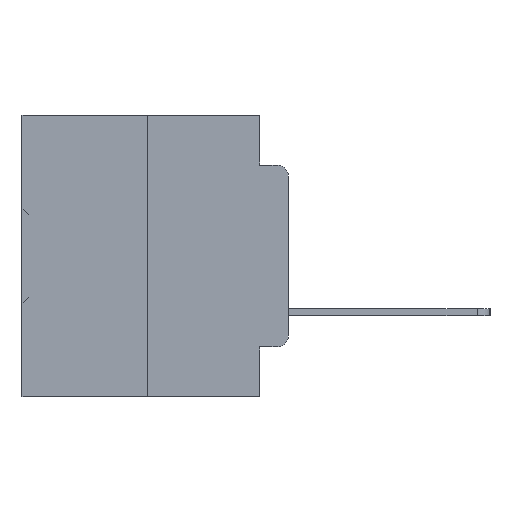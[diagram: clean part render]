
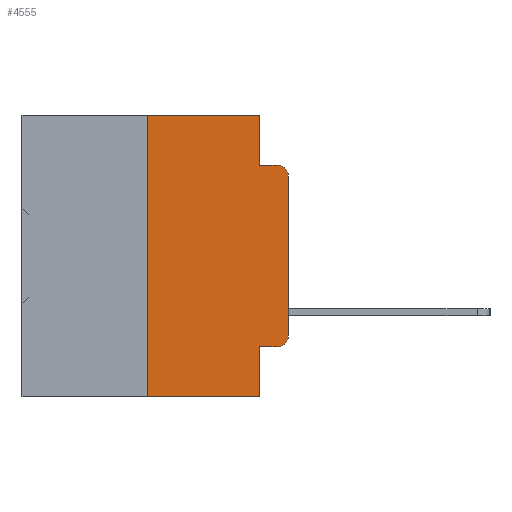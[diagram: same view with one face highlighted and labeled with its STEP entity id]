
A CAD part, left-side view. The second image highlights one B-rep face of the part: STEP entity #4555.
In plain terms, the highlighted planar face has unit normal (-1, 0, 0).
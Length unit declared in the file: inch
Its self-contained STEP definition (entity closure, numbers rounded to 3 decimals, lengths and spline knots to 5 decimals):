
#83 = CARTESIAN_POINT ( 'NONE',  ( 0., 0.25, -0.5 ) ) ;
#115 = CARTESIAN_POINT ( 'NONE',  ( 0., 0.051, -0.0885 ) ) ;
#621 = CARTESIAN_POINT ( 'NONE',  ( 0., 0.051, 0. ) ) ;
#1078 = DIRECTION ( 'NONE',  ( 0., 0., -1. ) ) ;
#1126 = DIRECTION ( 'NONE',  ( 1., 0., 0. ) ) ;
#1353 = CARTESIAN_POINT ( 'NONE',  ( 0., 0.02, -0.3915 ) ) ;
#2868 = CARTESIAN_POINT ( 'NONE',  ( 0., 0.051, -0.4115 ) ) ;
#3553 = CARTESIAN_POINT ( 'NONE',  ( 0., 0., -0.3915 ) ) ;
#3872 = ORIENTED_EDGE ( 'NONE', *, *, #26637, .F. ) ;
#4194 = FACE_OUTER_BOUND ( 'NONE', #36821, .T. ) ;
#4273 = DIRECTION ( 'NONE',  ( 0., 0., -1. ) ) ;
#4355 = DIRECTION ( 'NONE',  ( 0., -1., 0. ) ) ;
#4555 = ADVANCED_FACE ( 'NONE', ( #4194 ), #27442, .F. ) ;
#4786 = ORIENTED_EDGE ( 'NONE', *, *, #11222, .F. ) ;
#7142 = ORIENTED_EDGE ( 'NONE', *, *, #31402, .T. ) ;
#7289 = DIRECTION ( 'NONE',  ( 0., -1., 0. ) ) ;
#7305 = VECTOR ( 'NONE', #7289, 39.37008 ) ;
#7321 = EDGE_CURVE ( 'NONE', #8021, #9298, #30567, .T. ) ;
#7781 = VERTEX_POINT ( 'NONE', #17082 ) ;
#8021 = VERTEX_POINT ( 'NONE', #83 ) ;
#8659 = VERTEX_POINT ( 'NONE', #3553 ) ;
#8946 = VERTEX_POINT ( 'NONE', #2868 ) ;
#9113 = VECTOR ( 'NONE', #4355, 39.37008 ) ;
#9298 = VERTEX_POINT ( 'NONE', #10893 ) ;
#9777 = LINE ( 'NONE', #36849, #16595 ) ;
#10030 = LINE ( 'NONE', #32965, #9113 ) ;
#10893 = CARTESIAN_POINT ( 'NONE',  ( 0., 0.25, 0. ) ) ;
#11222 = EDGE_CURVE ( 'NONE', #16230, #32116, #18301, .T. ) ;
#11243 = DIRECTION ( 'NONE',  ( 0., 0., -1. ) ) ;
#11246 = ORIENTED_EDGE ( 'NONE', *, *, #7321, .F. ) ;
#11386 = CARTESIAN_POINT ( 'NONE',  ( 0., 0.02, -0.1085 ) ) ;
#12014 = AXIS2_PLACEMENT_3D ( 'NONE', #1353, #21587, #4273 ) ;
#12282 = ORIENTED_EDGE ( 'NONE', *, *, #34247, .T. ) ;
#12675 = CARTESIAN_POINT ( 'NONE',  ( 0., 0.051, 0. ) ) ;
#14001 = ORIENTED_EDGE ( 'NONE', *, *, #28544, .T. ) ;
#14309 = DIRECTION ( 'NONE',  ( 0., 0., -1. ) ) ;
#14568 = CARTESIAN_POINT ( 'NONE',  ( 0., 0.02, -0.0885 ) ) ;
#16230 = VERTEX_POINT ( 'NONE', #12675 ) ;
#16595 = VECTOR ( 'NONE', #11243, 39.37008 ) ;
#17082 = CARTESIAN_POINT ( 'NONE',  ( 0., 0.02, -0.4115 ) ) ;
#17598 = EDGE_CURVE ( 'NONE', #9298, #16230, #10030, .T. ) ;
#17795 = VERTEX_POINT ( 'NONE', #28285 ) ;
#18301 = LINE ( 'NONE', #621, #31707 ) ;
#19358 = DIRECTION ( 'NONE',  ( 0., 0., 1. ) ) ;
#19765 = VECTOR ( 'NONE', #19358, 39.37008 ) ;
#20023 = ORIENTED_EDGE ( 'NONE', *, *, #17598, .F. ) ;
#20386 = VECTOR ( 'NONE', #31371, 39.37008 ) ;
#20851 = DIRECTION ( 'NONE',  ( 0., 0., -1. ) ) ;
#21167 = LINE ( 'NONE', #35821, #27898 ) ;
#21258 = ORIENTED_EDGE ( 'NONE', *, *, #34949, .F. ) ;
#21281 = LINE ( 'NONE', #25665, #20386 ) ;
#21587 = DIRECTION ( 'NONE',  ( -1., 0., 0. ) ) ;
#22149 = VERTEX_POINT ( 'NONE', #14568 ) ;
#23080 = ORIENTED_EDGE ( 'NONE', *, *, #25427, .T. ) ;
#24493 = DIRECTION ( 'NONE',  ( 0., -1., 0. ) ) ;
#24547 = CARTESIAN_POINT ( 'NONE',  ( 0., 0.051, -0.4115 ) ) ;
#25427 = EDGE_CURVE ( 'NONE', #7781, #8659, #30842, .T. ) ;
#25665 = CARTESIAN_POINT ( 'NONE',  ( 0., 0.473, -0.5 ) ) ;
#26637 = EDGE_CURVE ( 'NONE', #32116, #22149, #21167, .T. ) ;
#27442 = PLANE ( 'NONE',  #29269 ) ;
#27898 = VECTOR ( 'NONE', #24493, 39.37008 ) ;
#28070 = CARTESIAN_POINT ( 'NONE',  ( 0., 0.473, 0. ) ) ;
#28285 = CARTESIAN_POINT ( 'NONE',  ( 0., 0.051, -0.5 ) ) ;
#28544 = EDGE_CURVE ( 'NONE', #32725, #22149, #37073, .T. ) ;
#29170 = LINE ( 'NONE', #33805, #19765 ) ;
#29269 = AXIS2_PLACEMENT_3D ( 'NONE', #28070, #1126, #1078 ) ;
#29324 = LINE ( 'NONE', #24547, #7305 ) ;
#30567 = LINE ( 'NONE', #36111, #37217 ) ;
#30842 = CIRCLE ( 'NONE', #12014, 0.02 ) ;
#31131 = EDGE_CURVE ( 'NONE', #8946, #7781, #29324, .T. ) ;
#31371 = DIRECTION ( 'NONE',  ( 0., -1., 0. ) ) ;
#31402 = EDGE_CURVE ( 'NONE', #8021, #17795, #21281, .T. ) ;
#31426 = DIRECTION ( 'NONE',  ( -1., 0., 0. ) ) ;
#31707 = VECTOR ( 'NONE', #20851, 39.37008 ) ;
#31769 = AXIS2_PLACEMENT_3D ( 'NONE', #11386, #31426, #14309 ) ;
#32116 = VERTEX_POINT ( 'NONE', #115 ) ;
#32725 = VERTEX_POINT ( 'NONE', #34780 ) ;
#32965 = CARTESIAN_POINT ( 'NONE',  ( 0., 0.473, 0. ) ) ;
#33632 = ORIENTED_EDGE ( 'NONE', *, *, #31131, .T. ) ;
#33805 = CARTESIAN_POINT ( 'NONE',  ( 0., 0., 0. ) ) ;
#34130 = DIRECTION ( 'NONE',  ( 0., 0., 1. ) ) ;
#34247 = EDGE_CURVE ( 'NONE', #8659, #32725, #29170, .T. ) ;
#34780 = CARTESIAN_POINT ( 'NONE',  ( 0., 0., -0.1085 ) ) ;
#34949 = EDGE_CURVE ( 'NONE', #8946, #17795, #9777, .T. ) ;
#35821 = CARTESIAN_POINT ( 'NONE',  ( 0., 0.051, -0.0885 ) ) ;
#36111 = CARTESIAN_POINT ( 'NONE',  ( 0., 0.25, 0. ) ) ;
#36821 = EDGE_LOOP ( 'NONE', ( #12282, #14001, #3872, #4786, #20023, #11246, #7142, #21258, #33632, #23080 ) ) ;
#36849 = CARTESIAN_POINT ( 'NONE',  ( 0., 0.051, 0. ) ) ;
#37073 = CIRCLE ( 'NONE', #31769, 0.02 ) ;
#37217 = VECTOR ( 'NONE', #34130, 39.37008 ) ;
